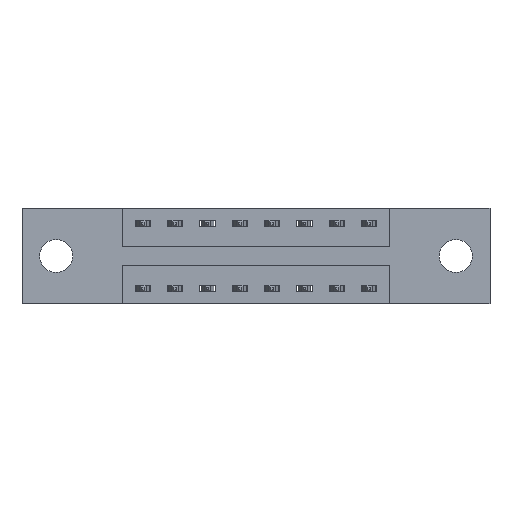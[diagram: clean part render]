
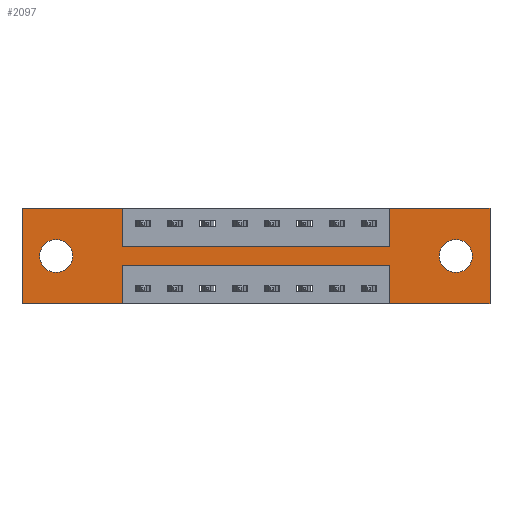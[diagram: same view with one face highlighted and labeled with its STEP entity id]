
A CAD part, front view. The second image highlights one B-rep face of the part: STEP entity #2097.
In plain terms, the highlighted planar face has unit normal (0, -1, 0).
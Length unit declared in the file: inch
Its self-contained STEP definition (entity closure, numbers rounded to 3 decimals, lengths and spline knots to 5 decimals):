
#53 = VERTEX_POINT ( 'NONE', #6479 ) ;
#97 = CARTESIAN_POINT ( 'NONE',  ( 0.3875, 0., 0. ) ) ;
#298 = ORIENTED_EDGE ( 'NONE', *, *, #3528, .F. ) ;
#337 = CIRCLE ( 'NONE', #2199, 0.064 ) ;
#486 = AXIS2_PLACEMENT_3D ( 'NONE', #7990, #3450, #4163 ) ;
#517 = VERTEX_POINT ( 'NONE', #8339 ) ;
#518 = CARTESIAN_POINT ( 'NONE',  ( 0., 0., -0.37 ) ) ;
#591 = FACE_OUTER_BOUND ( 'NONE', #9323, .T. ) ;
#716 = VERTEX_POINT ( 'NONE', #6227 ) ;
#763 = EDGE_CURVE ( 'NONE', #7075, #517, #9475, .T. ) ;
#864 = VECTOR ( 'NONE', #7866, 39.37008 ) ;
#994 = EDGE_LOOP ( 'NONE', ( #3036, #9807 ) ) ;
#1015 = EDGE_CURVE ( 'NONE', #7963, #4515, #4679, .T. ) ;
#1061 = CARTESIAN_POINT ( 'NONE',  ( 0., 0., 0. ) ) ;
#1119 = EDGE_CURVE ( 'NONE', #8406, #7341, #9820, .T. ) ;
#1342 = ORIENTED_EDGE ( 'NONE', *, *, #7318, .F. ) ;
#1574 = DIRECTION ( 'NONE',  ( 0., 0., 1. ) ) ;
#1621 = VECTOR ( 'NONE', #6953, 39.37008 ) ;
#1686 = EDGE_LOOP ( 'NONE', ( #7359, #2774 ) ) ;
#1718 = EDGE_CURVE ( 'NONE', #4515, #7963, #3611, .T. ) ;
#1734 = AXIS2_PLACEMENT_3D ( 'NONE', #8518, #7094, #7728 ) ;
#1779 = DIRECTION ( 'NONE',  ( 1., 0., 0. ) ) ;
#1818 = CARTESIAN_POINT ( 'NONE',  ( 1.4225, 0., -0.37 ) ) ;
#1874 = DIRECTION ( 'NONE',  ( 0., 1., 0. ) ) ;
#1975 = EDGE_CURVE ( 'NONE', #53, #8203, #6828, .T. ) ;
#1983 = VECTOR ( 'NONE', #1574, 39.37008 ) ;
#2042 = CARTESIAN_POINT ( 'NONE',  ( 0.3875, 0., -0.22 ) ) ;
#2097 = ADVANCED_FACE ( 'NONE', ( #9803, #3963, #591 ), #7849, .T. ) ;
#2199 = AXIS2_PLACEMENT_3D ( 'NONE', #4644, #4619, #7577 ) ;
#2298 = EDGE_CURVE ( 'NONE', #4929, #8151, #5823, .T. ) ;
#2438 = CARTESIAN_POINT ( 'NONE',  ( 1.4225, 0., -0.22 ) ) ;
#2501 = AXIS2_PLACEMENT_3D ( 'NONE', #5593, #5555, #5493 ) ;
#2597 = CARTESIAN_POINT ( 'NONE',  ( 1.81, 0., -0.37 ) ) ;
#2661 = CARTESIAN_POINT ( 'NONE',  ( 0., 0., -0.37 ) ) ;
#2774 = ORIENTED_EDGE ( 'NONE', *, *, #3519, .T. ) ;
#2827 = CARTESIAN_POINT ( 'NONE',  ( 0.3875, 0., -0.22 ) ) ;
#2865 = VECTOR ( 'NONE', #4298, 39.37008 ) ;
#2933 = ORIENTED_EDGE ( 'NONE', *, *, #4565, .F. ) ;
#2937 = LINE ( 'NONE', #3379, #5047 ) ;
#3036 = ORIENTED_EDGE ( 'NONE', *, *, #1015, .T. ) ;
#3106 = EDGE_CURVE ( 'NONE', #8151, #3974, #2937, .T. ) ;
#3168 = ORIENTED_EDGE ( 'NONE', *, *, #5024, .F. ) ;
#3256 = ORIENTED_EDGE ( 'NONE', *, *, #7417, .F. ) ;
#3371 = VECTOR ( 'NONE', #5309, 39.37008 ) ;
#3379 = CARTESIAN_POINT ( 'NONE',  ( 0.3875, 0., 0. ) ) ;
#3450 = DIRECTION ( 'NONE',  ( 0., 1., 0. ) ) ;
#3519 = EDGE_CURVE ( 'NONE', #517, #7075, #337, .T. ) ;
#3528 = EDGE_CURVE ( 'NONE', #8424, #8406, #9361, .T. ) ;
#3611 = CIRCLE ( 'NONE', #486, 0.064 ) ;
#3824 = LINE ( 'NONE', #8169, #2865 ) ;
#3861 = DIRECTION ( 'NONE',  ( 0., 0., -1. ) ) ;
#3906 = LINE ( 'NONE', #4599, #1983 ) ;
#3963 = FACE_BOUND ( 'NONE', #1686, .T. ) ;
#3974 = VERTEX_POINT ( 'NONE', #5134 ) ;
#3996 = ORIENTED_EDGE ( 'NONE', *, *, #2298, .F. ) ;
#4163 = DIRECTION ( 'NONE',  ( 0., 0., -1. ) ) ;
#4199 = VERTEX_POINT ( 'NONE', #9232 ) ;
#4298 = DIRECTION ( 'NONE',  ( 0., 0., 1. ) ) ;
#4471 = ORIENTED_EDGE ( 'NONE', *, *, #3106, .F. ) ;
#4515 = VERTEX_POINT ( 'NONE', #7432 ) ;
#4565 = EDGE_CURVE ( 'NONE', #716, #4199, #3824, .T. ) ;
#4599 = CARTESIAN_POINT ( 'NONE',  ( 0., 0., 0. ) ) ;
#4619 = DIRECTION ( 'NONE',  ( 0., 1., 0. ) ) ;
#4644 = CARTESIAN_POINT ( 'NONE',  ( 0.1325, 0., -0.185 ) ) ;
#4679 = CIRCLE ( 'NONE', #1734, 0.064 ) ;
#4929 = VERTEX_POINT ( 'NONE', #1061 ) ;
#4981 = CARTESIAN_POINT ( 'NONE',  ( 0.1325, 0., -0.185 ) ) ;
#5024 = EDGE_CURVE ( 'NONE', #8203, #7374, #7321, .T. ) ;
#5047 = VECTOR ( 'NONE', #9458, 39.37008 ) ;
#5134 = CARTESIAN_POINT ( 'NONE',  ( 0.3875, 0., -0.15 ) ) ;
#5135 = CARTESIAN_POINT ( 'NONE',  ( 0.3875, 0., -0.37 ) ) ;
#5231 = LINE ( 'NONE', #9184, #3371 ) ;
#5309 = DIRECTION ( 'NONE',  ( 1., 0., 0. ) ) ;
#5402 = EDGE_CURVE ( 'NONE', #7341, #4929, #3906, .T. ) ;
#5493 = DIRECTION ( 'NONE',  ( 0., 0., -1. ) ) ;
#5519 = VECTOR ( 'NONE', #8834, 39.37008 ) ;
#5555 = DIRECTION ( 'NONE',  ( 0., -1., 0. ) ) ;
#5557 = ORIENTED_EDGE ( 'NONE', *, *, #1119, .F. ) ;
#5593 = CARTESIAN_POINT ( 'NONE',  ( 0., 0., -0.37 ) ) ;
#5630 = CARTESIAN_POINT ( 'NONE',  ( 0.1325, 0., -0.121 ) ) ;
#5698 = CARTESIAN_POINT ( 'NONE',  ( 0., 0., 0. ) ) ;
#5823 = LINE ( 'NONE', #5698, #9622 ) ;
#5943 = CARTESIAN_POINT ( 'NONE',  ( 1.4225, 0., -0.37 ) ) ;
#6089 = LINE ( 'NONE', #7873, #7038 ) ;
#6133 = CARTESIAN_POINT ( 'NONE',  ( 1.6775, 0., -0.121 ) ) ;
#6227 = CARTESIAN_POINT ( 'NONE',  ( 1.4225, 0., -0.15 ) ) ;
#6370 = LINE ( 'NONE', #2042, #864 ) ;
#6374 = EDGE_CURVE ( 'NONE', #3974, #716, #6089, .T. ) ;
#6428 = EDGE_CURVE ( 'NONE', #7374, #7480, #7154, .T. ) ;
#6479 = CARTESIAN_POINT ( 'NONE',  ( 1.81, 0., 0. ) ) ;
#6539 = ORIENTED_EDGE ( 'NONE', *, *, #5402, .F. ) ;
#6645 = CARTESIAN_POINT ( 'NONE',  ( 1.81, 0., 0. ) ) ;
#6750 = ORIENTED_EDGE ( 'NONE', *, *, #6374, .F. ) ;
#6828 = LINE ( 'NONE', #6645, #8374 ) ;
#6953 = DIRECTION ( 'NONE',  ( 0., 0., -1. ) ) ;
#7038 = VECTOR ( 'NONE', #1779, 39.37008 ) ;
#7075 = VERTEX_POINT ( 'NONE', #5630 ) ;
#7094 = DIRECTION ( 'NONE',  ( 0., 1., 0. ) ) ;
#7154 = LINE ( 'NONE', #1818, #7262 ) ;
#7202 = ORIENTED_EDGE ( 'NONE', *, *, #1975, .F. ) ;
#7262 = VECTOR ( 'NONE', #7900, 39.37008 ) ;
#7318 = EDGE_CURVE ( 'NONE', #7480, #8424, #6370, .T. ) ;
#7321 = LINE ( 'NONE', #518, #5519 ) ;
#7341 = VERTEX_POINT ( 'NONE', #8167 ) ;
#7347 = AXIS2_PLACEMENT_3D ( 'NONE', #4981, #1874, #8848 ) ;
#7359 = ORIENTED_EDGE ( 'NONE', *, *, #763, .T. ) ;
#7374 = VERTEX_POINT ( 'NONE', #5943 ) ;
#7417 = EDGE_CURVE ( 'NONE', #4199, #53, #5231, .T. ) ;
#7432 = CARTESIAN_POINT ( 'NONE',  ( 1.6775, 0., -0.249 ) ) ;
#7480 = VERTEX_POINT ( 'NONE', #2438 ) ;
#7577 = DIRECTION ( 'NONE',  ( 0., 0., 1. ) ) ;
#7728 = DIRECTION ( 'NONE',  ( 0., 0., -1. ) ) ;
#7849 = PLANE ( 'NONE',  #2501 ) ;
#7866 = DIRECTION ( 'NONE',  ( -1., 0., 0. ) ) ;
#7873 = CARTESIAN_POINT ( 'NONE',  ( 0.3875, 0., -0.15 ) ) ;
#7900 = DIRECTION ( 'NONE',  ( 0., 0., 1. ) ) ;
#7963 = VERTEX_POINT ( 'NONE', #6133 ) ;
#7990 = CARTESIAN_POINT ( 'NONE',  ( 1.6775, 0., -0.185 ) ) ;
#8012 = ORIENTED_EDGE ( 'NONE', *, *, #6428, .F. ) ;
#8020 = DIRECTION ( 'NONE',  ( -1., 0., 0. ) ) ;
#8151 = VERTEX_POINT ( 'NONE', #97 ) ;
#8167 = CARTESIAN_POINT ( 'NONE',  ( 0., 0., -0.37 ) ) ;
#8169 = CARTESIAN_POINT ( 'NONE',  ( 1.4225, 0., 0. ) ) ;
#8203 = VERTEX_POINT ( 'NONE', #2597 ) ;
#8339 = CARTESIAN_POINT ( 'NONE',  ( 0.1325, 0., -0.249 ) ) ;
#8374 = VECTOR ( 'NONE', #3861, 39.37008 ) ;
#8406 = VERTEX_POINT ( 'NONE', #5135 ) ;
#8424 = VERTEX_POINT ( 'NONE', #2827 ) ;
#8444 = CARTESIAN_POINT ( 'NONE',  ( 0.3875, 0., -0.37 ) ) ;
#8518 = CARTESIAN_POINT ( 'NONE',  ( 1.6775, 0., -0.185 ) ) ;
#8834 = DIRECTION ( 'NONE',  ( -1., 0., 0. ) ) ;
#8848 = DIRECTION ( 'NONE',  ( 0., 0., 1. ) ) ;
#9184 = CARTESIAN_POINT ( 'NONE',  ( 0., 0., 0. ) ) ;
#9232 = CARTESIAN_POINT ( 'NONE',  ( 1.4225, 0., 0. ) ) ;
#9323 = EDGE_LOOP ( 'NONE', ( #298, #1342, #8012, #3168, #7202, #3256, #2933, #6750, #4471, #3996, #6539, #5557 ) ) ;
#9361 = LINE ( 'NONE', #8444, #1621 ) ;
#9458 = DIRECTION ( 'NONE',  ( 0., 0., -1. ) ) ;
#9475 = CIRCLE ( 'NONE', #7347, 0.064 ) ;
#9622 = VECTOR ( 'NONE', #9721, 39.37008 ) ;
#9701 = VECTOR ( 'NONE', #8020, 39.37008 ) ;
#9721 = DIRECTION ( 'NONE',  ( 1., 0., 0. ) ) ;
#9803 = FACE_BOUND ( 'NONE', #994, .T. ) ;
#9807 = ORIENTED_EDGE ( 'NONE', *, *, #1718, .T. ) ;
#9820 = LINE ( 'NONE', #2661, #9701 ) ;
